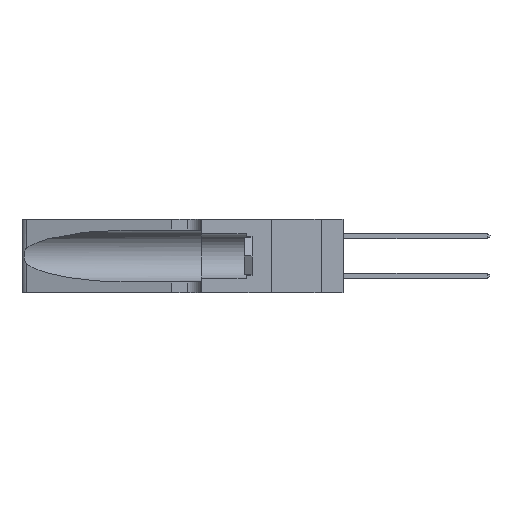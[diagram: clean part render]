
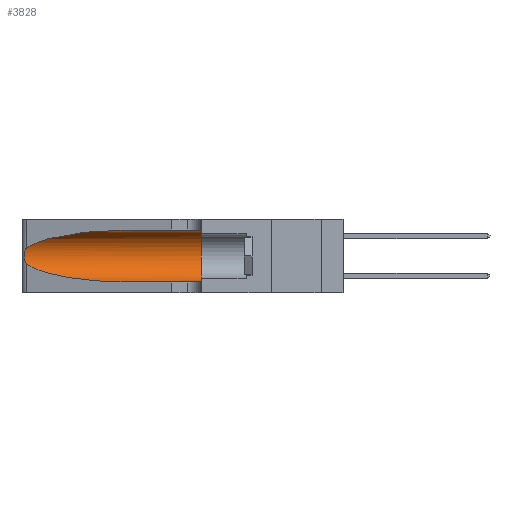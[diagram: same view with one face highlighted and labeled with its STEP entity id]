
A CAD part, left-side view. The second image highlights one B-rep face of the part: STEP entity #3828.
In plain terms, the highlighted cylindrical face has radius 3.308 mm (diameter 6.617 mm), a partial arc.
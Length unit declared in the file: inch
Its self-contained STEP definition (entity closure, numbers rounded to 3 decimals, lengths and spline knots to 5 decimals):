
#18 = ORIENTED_EDGE ( 'NONE', *, *, #36868, .T. ) ;
#1338 = B_SPLINE_CURVE_WITH_KNOTS ( 'NONE', 3,
 ( #16873, #37906, #21010, #2039, #30896, #11351, #21450, #14500, #8493, #1465, #8364, #21163, #15088, #34312 ),
 .UNSPECIFIED., .F., .F.,
 ( 4, 2, 2, 2, 2, 2, 4 ),
 ( 0., 0.00027, 0.00053, 0.00107, 0.0016, 0.00187, 0.00214 ),
 .UNSPECIFIED. ) ;
#1430 = LINE ( 'NONE', #15307, #35180 ) ;
#1465 = CARTESIAN_POINT ( 'NONE',  ( 0.25856, 1.23593, 0.16098 ) ) ;
#2039 = CARTESIAN_POINT ( 'NONE',  ( 0.25787, 1.23484, 0.2124 ) ) ;
#3807 = CARTESIAN_POINT ( 'NONE',  ( 0.1305, 1.61858, 0.185 ) ) ;
#3828 = ADVANCED_FACE ( 'NONE', ( #20038 ), #19063, .F. ) ;
#5255 = CARTESIAN_POINT ( 'NONE',  ( 0.25487, 1.22718, 0.14631 ) ) ;
#6045 = VERTEX_POINT ( 'NONE', #37734 ) ;
#7613 = VERTEX_POINT ( 'NONE', #5255 ) ;
#7857 = EDGE_CURVE ( 'NONE', #19618, #6045, #28859, .T. ) ;
#8364 = CARTESIAN_POINT ( 'NONE',  ( 0.25789, 1.23486, 0.15765 ) ) ;
#8493 = CARTESIAN_POINT ( 'NONE',  ( 0.26017, 1.23833, 0.17102 ) ) ;
#8790 = ORIENTED_EDGE ( 'NONE', *, *, #23087, .T. ) ;
#9804 = ORIENTED_EDGE ( 'NONE', *, *, #35399, .T. ) ;
#10009 = CARTESIAN_POINT ( 'NONE',  ( 0.25487, 1.22718, 0.22369 ) ) ;
#10418 = DIRECTION ( 'NONE',  ( 0., -1., 0. ) ) ;
#11118 = CARTESIAN_POINT ( 'NONE',  ( 0.2373, 1.15595, 0.28018 ) ) ;
#11351 = CARTESIAN_POINT ( 'NONE',  ( 0.26018, 1.23835, 0.19895 ) ) ;
#11771 = VERTEX_POINT ( 'NONE', #38131 ) ;
#13713 = EDGE_CURVE ( 'NONE', #18288, #37340, #22807, .T. ) ;
#14208 = CARTESIAN_POINT ( 'NONE',  ( 0.25487, 1.22718, 0.14631 ) ) ;
#14409 = VECTOR ( 'NONE', #28001, 39.37008 ) ;
#14500 = CARTESIAN_POINT ( 'NONE',  ( 0.26075, 1.23896, 0.178 ) ) ;
#14712 = CARTESIAN_POINT ( 'NONE',  ( 0.25487, 1.22718, 0.22369 ) ) ;
#15088 = CARTESIAN_POINT ( 'NONE',  ( 0.25555, 1.22993, 0.14849 ) ) ;
#15307 = CARTESIAN_POINT ( 'NONE',  ( 0.1305, 1.61858, 0.05475 ) ) ;
#16873 = CARTESIAN_POINT ( 'NONE',  ( 0.25487, 1.22718, 0.22369 ) ) ;
#16886 = CARTESIAN_POINT ( 'NONE',  ( 0.1305, 0.72297, 0.31525 ) ) ;
#17341 = CARTESIAN_POINT ( 'NONE',  ( 0.18966, 0.96281, 0.05475 ) ) ;
#18284 = EDGE_LOOP ( 'NONE', ( #21575, #18, #8790, #9804, #31142, #29868 ) ) ;
#18288 = VERTEX_POINT ( 'NONE', #16886 ) ;
#19063 = CYLINDRICAL_SURFACE ( 'NONE', #37687, 0.13025 ) ;
#19618 = VERTEX_POINT ( 'NONE', #37717 ) ;
#20038 = FACE_OUTER_BOUND ( 'NONE', #18284, .T. ) ;
#20298 = CARTESIAN_POINT ( 'NONE',  ( 0.1305, 0.72297, 0.05475 ) ) ;
#21010 = CARTESIAN_POINT ( 'NONE',  ( 0.25639, 1.23184, 0.21858 ) ) ;
#21163 = CARTESIAN_POINT ( 'NONE',  ( 0.25639, 1.23186, 0.15144 ) ) ;
#21450 = CARTESIAN_POINT ( 'NONE',  ( 0.26075, 1.23896, 0.19203 ) ) ;
#21575 = ORIENTED_EDGE ( 'NONE', *, *, #13713, .T. ) ;
#22807 =( BOUNDED_CURVE ( )  B_SPLINE_CURVE ( 3, ( #36935, #37076, #11118, #14712 ),
 .UNSPECIFIED., .F., .T. ) 
 B_SPLINE_CURVE_WITH_KNOTS ( ( 4, 4 ),
 ( 1.5708, 2.84003 ),
 .UNSPECIFIED. ) 
 CURVE ( )  GEOMETRIC_REPRESENTATION_ITEM ( )  RATIONAL_B_SPLINE_CURVE ( ( 1., 0.87, 0.87, 1. ) ) 
 REPRESENTATION_ITEM ( '' )  );
#23087 = EDGE_CURVE ( 'NONE', #7613, #11771, #37486, .T. ) ;
#26821 = DIRECTION ( 'NONE',  ( 0., 0., -1. ) ) ;
#28001 = DIRECTION ( 'NONE',  ( 0., -1., 0. ) ) ;
#28859 = CIRCLE ( 'NONE', #33320, 0.13025 ) ;
#29440 = DIRECTION ( 'NONE',  ( 0., 0., 1. ) ) ;
#29868 = ORIENTED_EDGE ( 'NONE', *, *, #33442, .F. ) ;
#30896 = CARTESIAN_POINT ( 'NONE',  ( 0.25854, 1.2359, 0.20912 ) ) ;
#31142 = ORIENTED_EDGE ( 'NONE', *, *, #7857, .F. ) ;
#33320 = AXIS2_PLACEMENT_3D ( 'NONE', #35445, #39139, #29440 ) ;
#33442 = EDGE_CURVE ( 'NONE', #18288, #19618, #41479, .T. ) ;
#34312 = CARTESIAN_POINT ( 'NONE',  ( 0.25487, 1.22718, 0.14631 ) ) ;
#35180 = VECTOR ( 'NONE', #35957, 39.37008 ) ;
#35399 = EDGE_CURVE ( 'NONE', #11771, #6045, #1430, .T. ) ;
#35445 = CARTESIAN_POINT ( 'NONE',  ( 0.1305, 0.35, 0.185 ) ) ;
#35957 = DIRECTION ( 'NONE',  ( 0., -1., 0. ) ) ;
#36868 = EDGE_CURVE ( 'NONE', #37340, #7613, #1338, .T. ) ;
#36897 = CARTESIAN_POINT ( 'NONE',  ( 0.2373, 1.15595, 0.08982 ) ) ;
#36935 = CARTESIAN_POINT ( 'NONE',  ( 0.1305, 0.72297, 0.31525 ) ) ;
#37076 = CARTESIAN_POINT ( 'NONE',  ( 0.18966, 0.96281, 0.31525 ) ) ;
#37340 = VERTEX_POINT ( 'NONE', #10009 ) ;
#37486 =( BOUNDED_CURVE ( )  B_SPLINE_CURVE ( 3, ( #14208, #36897, #17341, #20298 ),
 .UNSPECIFIED., .F., .T. ) 
 B_SPLINE_CURVE_WITH_KNOTS ( ( 4, 4 ),
 ( 3.44316, 4.71239 ),
 .UNSPECIFIED. ) 
 CURVE ( )  GEOMETRIC_REPRESENTATION_ITEM ( )  RATIONAL_B_SPLINE_CURVE ( ( 1., 0.87, 0.87, 1. ) ) 
 REPRESENTATION_ITEM ( '' )  );
#37687 = AXIS2_PLACEMENT_3D ( 'NONE', #3807, #10418, #26821 ) ;
#37717 = CARTESIAN_POINT ( 'NONE',  ( 0.1305, 0.35, 0.31525 ) ) ;
#37734 = CARTESIAN_POINT ( 'NONE',  ( 0.1305, 0.35, 0.05475 ) ) ;
#37906 = CARTESIAN_POINT ( 'NONE',  ( 0.25555, 1.22994, 0.2215 ) ) ;
#37941 = CARTESIAN_POINT ( 'NONE',  ( 0.1305, 1.61858, 0.31525 ) ) ;
#38131 = CARTESIAN_POINT ( 'NONE',  ( 0.1305, 0.72297, 0.05475 ) ) ;
#39139 = DIRECTION ( 'NONE',  ( 0., 1., 0. ) ) ;
#41479 = LINE ( 'NONE', #37941, #14409 ) ;
